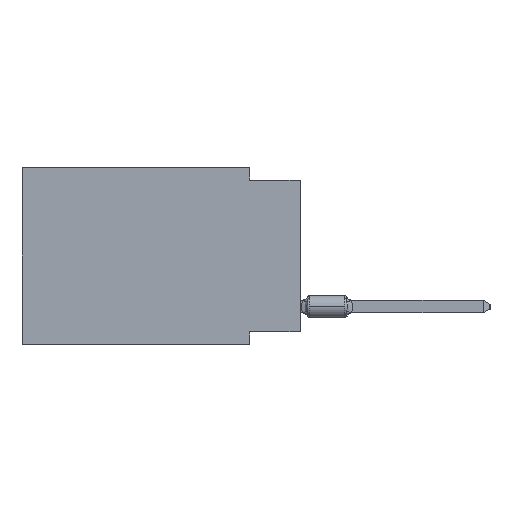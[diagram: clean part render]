
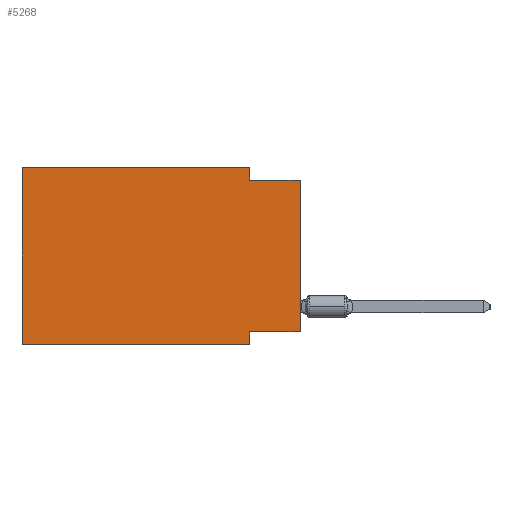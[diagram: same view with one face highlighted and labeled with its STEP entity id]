
A CAD part, left-side view. The second image highlights one B-rep face of the part: STEP entity #5268.
In plain terms, the highlighted planar face has unit normal (-1, 0, 0).
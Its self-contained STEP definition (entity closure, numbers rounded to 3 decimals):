
#220 = DIRECTION ( 'NONE',  ( 0., -1., 0. ) ) ;
#1347 = CARTESIAN_POINT ( 'NONE',  ( 0., 0., -0.635 ) ) ;
#1540 = LINE ( 'NONE', #73656, #88471 ) ;
#2415 = EDGE_CURVE ( 'NONE', #83894, #24311, #36311, .T. ) ;
#2615 = DIRECTION ( 'NONE',  ( 1., 0., 0. ) ) ;
#3465 = EDGE_CURVE ( 'NONE', #21730, #12191, #96233, .T. ) ;
#3498 = EDGE_CURVE ( 'NONE', #38088, #25631, #72869, .T. ) ;
#3677 = CARTESIAN_POINT ( 'NONE',  ( 0., 2.54, -8.89 ) ) ;
#5268 = ADVANCED_FACE ( 'NONE', ( #89293 ), #10396, .F. ) ;
#6031 = VECTOR ( 'NONE', #32049, 1000. ) ;
#7227 = LINE ( 'NONE', #36810, #25466 ) ;
#7796 = EDGE_CURVE ( 'NONE', #83894, #12191, #24666, .T. ) ;
#9732 = CARTESIAN_POINT ( 'NONE',  ( 0., 2.54, -0.635 ) ) ;
#9843 = DIRECTION ( 'NONE',  ( 0., 0., 1. ) ) ;
#10396 = PLANE ( 'NONE',  #76490 ) ;
#11439 = DIRECTION ( 'NONE',  ( 0., 1., 0. ) ) ;
#11636 = LINE ( 'NONE', #70983, #6031 ) ;
#12191 = VERTEX_POINT ( 'NONE', #1347 ) ;
#15978 = EDGE_LOOP ( 'NONE', ( #58812, #74822, #57745, #82175, #101393, #79643, #33092, #80102 ) ) ;
#21321 = EDGE_CURVE ( 'NONE', #50873, #38088, #1540, .T. ) ;
#21730 = VERTEX_POINT ( 'NONE', #9732 ) ;
#24311 = VERTEX_POINT ( 'NONE', #77260 ) ;
#24666 = LINE ( 'NONE', #26188, #93449 ) ;
#25466 = VECTOR ( 'NONE', #86102, 1000. ) ;
#25631 = VERTEX_POINT ( 'NONE', #45934 ) ;
#26188 = CARTESIAN_POINT ( 'NONE',  ( 0., 0., 0. ) ) ;
#31524 = VECTOR ( 'NONE', #34447, 1000. ) ;
#32049 = DIRECTION ( 'NONE',  ( 0., 0., -1. ) ) ;
#33092 = ORIENTED_EDGE ( 'NONE', *, *, #76080, .F. ) ;
#34264 = DIRECTION ( 'NONE',  ( 0., 0., -1. ) ) ;
#34447 = DIRECTION ( 'NONE',  ( 0., -1., 0. ) ) ;
#34992 = EDGE_CURVE ( 'NONE', #50873, #77189, #66836, .T. ) ;
#36311 = LINE ( 'NONE', #81167, #62793 ) ;
#36810 = CARTESIAN_POINT ( 'NONE',  ( 0., 2.54, -8.89 ) ) ;
#37887 = CARTESIAN_POINT ( 'NONE',  ( 0., 13.97, -8.89 ) ) ;
#38046 = VECTOR ( 'NONE', #220, 1000. ) ;
#38088 = VERTEX_POINT ( 'NONE', #49514 ) ;
#42029 = CARTESIAN_POINT ( 'NONE',  ( 0., 13.97, 0. ) ) ;
#45934 = CARTESIAN_POINT ( 'NONE',  ( 0., 2.54, 0. ) ) ;
#49514 = CARTESIAN_POINT ( 'NONE',  ( 0., 13.97, 0. ) ) ;
#50249 = CARTESIAN_POINT ( 'NONE',  ( 0., 13.97, -8.89 ) ) ;
#50873 = VERTEX_POINT ( 'NONE', #37887 ) ;
#54701 = CARTESIAN_POINT ( 'NONE',  ( 0., 0., -0.635 ) ) ;
#56812 = DIRECTION ( 'NONE',  ( 0., 0., 1. ) ) ;
#57745 = ORIENTED_EDGE ( 'NONE', *, *, #81727, .F. ) ;
#58812 = ORIENTED_EDGE ( 'NONE', *, *, #7796, .T. ) ;
#59058 = DIRECTION ( 'NONE',  ( 0., -1., 0. ) ) ;
#62793 = VECTOR ( 'NONE', #11439, 1000. ) ;
#66836 = LINE ( 'NONE', #50249, #69786 ) ;
#69786 = VECTOR ( 'NONE', #59058, 1000. ) ;
#70983 = CARTESIAN_POINT ( 'NONE',  ( 0., 2.54, 0. ) ) ;
#72869 = LINE ( 'NONE', #88964, #31524 ) ;
#73656 = CARTESIAN_POINT ( 'NONE',  ( 0., 13.97, 0. ) ) ;
#74822 = ORIENTED_EDGE ( 'NONE', *, *, #3465, .F. ) ;
#76080 = EDGE_CURVE ( 'NONE', #24311, #77189, #7227, .T. ) ;
#76490 = AXIS2_PLACEMENT_3D ( 'NONE', #42029, #2615, #34264 ) ;
#77189 = VERTEX_POINT ( 'NONE', #3677 ) ;
#77260 = CARTESIAN_POINT ( 'NONE',  ( 0., 2.54, -8.255 ) ) ;
#79643 = ORIENTED_EDGE ( 'NONE', *, *, #34992, .T. ) ;
#80102 = ORIENTED_EDGE ( 'NONE', *, *, #2415, .F. ) ;
#80885 = CARTESIAN_POINT ( 'NONE',  ( 0., 0., -8.255 ) ) ;
#81167 = CARTESIAN_POINT ( 'NONE',  ( 0., 0., -8.255 ) ) ;
#81727 = EDGE_CURVE ( 'NONE', #25631, #21730, #11636, .T. ) ;
#82175 = ORIENTED_EDGE ( 'NONE', *, *, #3498, .F. ) ;
#83894 = VERTEX_POINT ( 'NONE', #80885 ) ;
#86102 = DIRECTION ( 'NONE',  ( 0., 0., -1. ) ) ;
#88471 = VECTOR ( 'NONE', #9843, 1000. ) ;
#88964 = CARTESIAN_POINT ( 'NONE',  ( 0., 13.97, 0. ) ) ;
#89293 = FACE_OUTER_BOUND ( 'NONE', #15978, .T. ) ;
#93449 = VECTOR ( 'NONE', #56812, 1000. ) ;
#96233 = LINE ( 'NONE', #54701, #38046 ) ;
#101393 = ORIENTED_EDGE ( 'NONE', *, *, #21321, .F. ) ;
